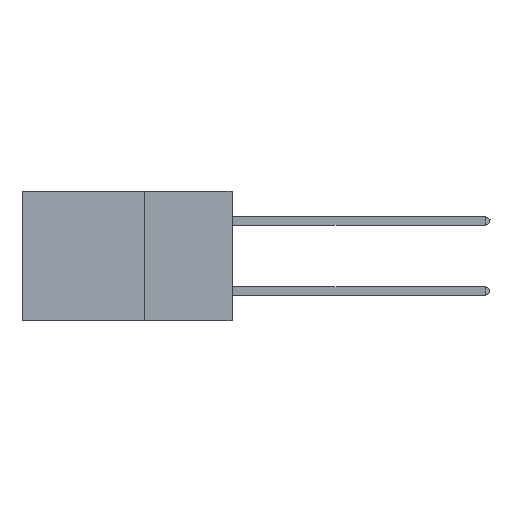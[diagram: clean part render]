
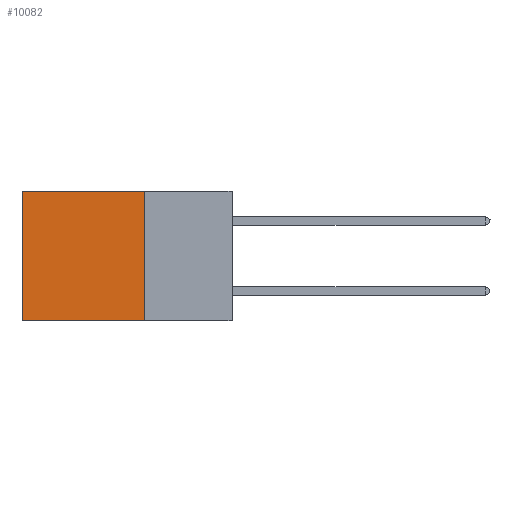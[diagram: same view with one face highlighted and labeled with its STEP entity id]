
A CAD part, left-side view. The second image highlights one B-rep face of the part: STEP entity #10082.
In plain terms, the highlighted planar face has unit normal (-1, 0, 0).
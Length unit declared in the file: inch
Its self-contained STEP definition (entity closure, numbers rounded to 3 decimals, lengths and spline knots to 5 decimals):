
#140 = CARTESIAN_POINT ( 'NONE',  ( 0.2875, 0.25, 0. ) ) ;
#178 = CARTESIAN_POINT ( 'NONE',  ( 0.2875, 0.6, 0. ) ) ;
#1013 = VERTEX_POINT ( 'NONE', #20514 ) ;
#1929 = PLANE ( 'NONE',  #26611 ) ;
#2721 = CARTESIAN_POINT ( 'NONE',  ( 0.2875, 0.25, 0. ) ) ;
#2756 = DIRECTION ( 'NONE',  ( 0., 0., -1. ) ) ;
#5072 = VERTEX_POINT ( 'NONE', #28713 ) ;
#6524 = ORIENTED_EDGE ( 'NONE', *, *, #31521, .F. ) ;
#8732 = VECTOR ( 'NONE', #30636, 39.37008 ) ;
#9672 = FACE_OUTER_BOUND ( 'NONE', #21840, .T. ) ;
#9997 = DIRECTION ( 'NONE',  ( 0., 1., 0. ) ) ;
#10082 = ADVANCED_FACE ( 'NONE', ( #9672 ), #1929, .F. ) ;
#10107 = CARTESIAN_POINT ( 'NONE',  ( 0.2875, 0.25, 0. ) ) ;
#10337 = LINE ( 'NONE', #178, #21746 ) ;
#11410 = CARTESIAN_POINT ( 'NONE',  ( 0.2875, 0.25, -0.37 ) ) ;
#11889 = VERTEX_POINT ( 'NONE', #10107 ) ;
#12743 = LINE ( 'NONE', #2721, #13892 ) ;
#12766 = EDGE_CURVE ( 'NONE', #22336, #5072, #10337, .T. ) ;
#12948 = ORIENTED_EDGE ( 'NONE', *, *, #25867, .T. ) ;
#13834 = LINE ( 'NONE', #11410, #8732 ) ;
#13892 = VECTOR ( 'NONE', #29543, 39.37008 ) ;
#14391 = ORIENTED_EDGE ( 'NONE', *, *, #17846, .F. ) ;
#15225 = ORIENTED_EDGE ( 'NONE', *, *, #12766, .T. ) ;
#17846 = EDGE_CURVE ( 'NONE', #1013, #5072, #13834, .T. ) ;
#19232 = CARTESIAN_POINT ( 'NONE',  ( 0.2875, 0.25, 0. ) ) ;
#20514 = CARTESIAN_POINT ( 'NONE',  ( 0.2875, 0.25, -0.37 ) ) ;
#21746 = VECTOR ( 'NONE', #2756, 39.37008 ) ;
#21840 = EDGE_LOOP ( 'NONE', ( #15225, #14391, #6524, #12948 ) ) ;
#22336 = VERTEX_POINT ( 'NONE', #30996 ) ;
#25867 = EDGE_CURVE ( 'NONE', #11889, #22336, #29234, .T. ) ;
#26611 = AXIS2_PLACEMENT_3D ( 'NONE', #19232, #29062, #29378 ) ;
#28081 = VECTOR ( 'NONE', #9997, 39.37008 ) ;
#28713 = CARTESIAN_POINT ( 'NONE',  ( 0.2875, 0.6, -0.37 ) ) ;
#29062 = DIRECTION ( 'NONE',  ( 1., 0., 0. ) ) ;
#29234 = LINE ( 'NONE', #140, #28081 ) ;
#29378 = DIRECTION ( 'NONE',  ( 0., 0., -1. ) ) ;
#29543 = DIRECTION ( 'NONE',  ( 0., 0., -1. ) ) ;
#30636 = DIRECTION ( 'NONE',  ( 0., 1., 0. ) ) ;
#30996 = CARTESIAN_POINT ( 'NONE',  ( 0.2875, 0.6, 0. ) ) ;
#31521 = EDGE_CURVE ( 'NONE', #11889, #1013, #12743, .T. ) ;
